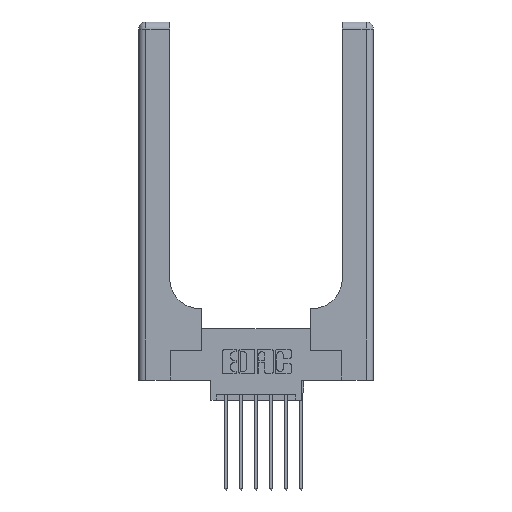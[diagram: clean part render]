
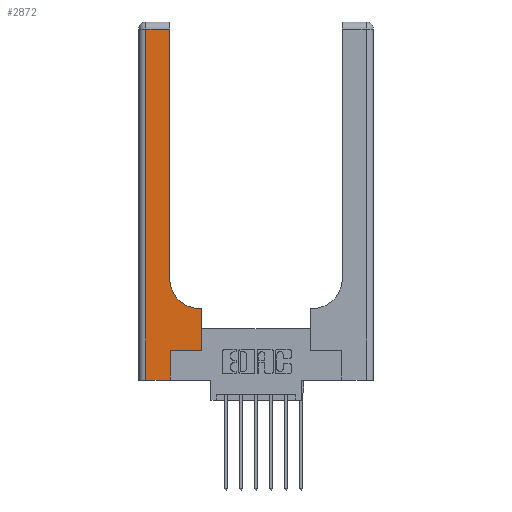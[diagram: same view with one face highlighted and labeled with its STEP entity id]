
A CAD part, top view. The second image highlights one B-rep face of the part: STEP entity #2872.
In plain terms, the highlighted planar face has unit normal (0, 0, 1).
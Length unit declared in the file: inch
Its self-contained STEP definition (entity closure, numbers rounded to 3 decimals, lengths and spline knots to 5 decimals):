
#15 = ORIENTED_EDGE ( 'NONE', *, *, #273, .T. ) ;
#273 = EDGE_CURVE ( 'NONE', #9280, #6992, #13074, .T. ) ;
#305 = AXIS2_PLACEMENT_3D ( 'NONE', #10387, #13940, #13862 ) ;
#487 = ORIENTED_EDGE ( 'NONE', *, *, #3870, .T. ) ;
#615 = LINE ( 'NONE', #5942, #1135 ) ;
#1119 = VERTEX_POINT ( 'NONE', #5577 ) ;
#1135 = VECTOR ( 'NONE', #10319, 39.37008 ) ;
#1679 = LINE ( 'NONE', #11591, #10200 ) ;
#1754 = VECTOR ( 'NONE', #6185, 39.37008 ) ;
#2082 = CARTESIAN_POINT ( 'NONE',  ( 0., 2.94, 0.37 ) ) ;
#2100 = DIRECTION ( 'NONE',  ( 1., 0., 0. ) ) ;
#2111 = CARTESIAN_POINT ( 'NONE',  ( 0.265, 0., 0.37 ) ) ;
#2166 = EDGE_CURVE ( 'NONE', #2642, #12599, #1679, .T. ) ;
#2642 = VERTEX_POINT ( 'NONE', #14012 ) ;
#2648 = VECTOR ( 'NONE', #4425, 39.37008 ) ;
#2872 = ADVANCED_FACE ( 'NONE', ( #6914 ), #4704, .F. ) ;
#2896 = AXIS2_PLACEMENT_3D ( 'NONE', #3637, #11289, #4423 ) ;
#3637 = CARTESIAN_POINT ( 'NONE',  ( 0., 3., 0.37 ) ) ;
#3650 = ORIENTED_EDGE ( 'NONE', *, *, #7391, .T. ) ;
#3870 = EDGE_CURVE ( 'NONE', #4499, #9280, #8801, .T. ) ;
#4423 = DIRECTION ( 'NONE',  ( -1., 0., 0. ) ) ;
#4425 = DIRECTION ( 'NONE',  ( -1., 0., 0. ) ) ;
#4499 = VERTEX_POINT ( 'NONE', #10076 ) ;
#4564 = EDGE_CURVE ( 'NONE', #12599, #7520, #9417, .T. ) ;
#4704 = PLANE ( 'NONE',  #2896 ) ;
#4987 = CARTESIAN_POINT ( 'NONE',  ( 0.06, 2.94, 0.37 ) ) ;
#5164 = CARTESIAN_POINT ( 'NONE',  ( 0., 0., 0.37 ) ) ;
#5577 = CARTESIAN_POINT ( 'NONE',  ( 0.51, 0.6, 0.37 ) ) ;
#5881 = CARTESIAN_POINT ( 'NONE',  ( 0.06, 0., 0.37 ) ) ;
#5942 = CARTESIAN_POINT ( 'NONE',  ( 0.26, 3., 0.37 ) ) ;
#6185 = DIRECTION ( 'NONE',  ( 0., 1., 0. ) ) ;
#6188 = LINE ( 'NONE', #7118, #6389 ) ;
#6356 = CARTESIAN_POINT ( 'NONE',  ( 0.26, 0.85, 0.37 ) ) ;
#6359 = CARTESIAN_POINT ( 'NONE',  ( 0.528, 0.6, 0.37 ) ) ;
#6389 = VECTOR ( 'NONE', #8336, 39.37008 ) ;
#6428 = CIRCLE ( 'NONE', #305, 0.25 ) ;
#6914 = FACE_OUTER_BOUND ( 'NONE', #9129, .T. ) ;
#6992 = VERTEX_POINT ( 'NONE', #5881 ) ;
#7118 = CARTESIAN_POINT ( 'NONE',  ( 0.26, 0.6, 0.37 ) ) ;
#7391 = EDGE_CURVE ( 'NONE', #13754, #4499, #615, .T. ) ;
#7520 = VERTEX_POINT ( 'NONE', #6359 ) ;
#7649 = EDGE_CURVE ( 'NONE', #13379, #2642, #9729, .T. ) ;
#8278 = EDGE_CURVE ( 'NONE', #6992, #13379, #11673, .T. ) ;
#8336 = DIRECTION ( 'NONE',  ( -1., 0., 0. ) ) ;
#8801 = LINE ( 'NONE', #2082, #2648 ) ;
#9129 = EDGE_LOOP ( 'NONE', ( #3650, #487, #15, #13179, #10462, #10946, #13648, #10937, #11899 ) ) ;
#9280 = VERTEX_POINT ( 'NONE', #4987 ) ;
#9417 = LINE ( 'NONE', #12411, #1754 ) ;
#9571 = VECTOR ( 'NONE', #9949, 39.37008 ) ;
#9729 = LINE ( 'NONE', #13019, #9571 ) ;
#9949 = DIRECTION ( 'NONE',  ( 0., 1., 0. ) ) ;
#10076 = CARTESIAN_POINT ( 'NONE',  ( 0.26, 2.94, 0.37 ) ) ;
#10200 = VECTOR ( 'NONE', #12539, 39.37008 ) ;
#10319 = DIRECTION ( 'NONE',  ( 0., 1., 0. ) ) ;
#10387 = CARTESIAN_POINT ( 'NONE',  ( 0.51, 0.85, 0.37 ) ) ;
#10462 = ORIENTED_EDGE ( 'NONE', *, *, #7649, .T. ) ;
#10686 = EDGE_CURVE ( 'NONE', #7520, #1119, #6188, .T. ) ;
#10937 = ORIENTED_EDGE ( 'NONE', *, *, #10686, .T. ) ;
#10946 = ORIENTED_EDGE ( 'NONE', *, *, #2166, .T. ) ;
#11289 = DIRECTION ( 'NONE',  ( 0., 0., -1. ) ) ;
#11506 = CARTESIAN_POINT ( 'NONE',  ( 0.528, 0.25, 0.37 ) ) ;
#11591 = CARTESIAN_POINT ( 'NONE',  ( 0.265, 0.25, 0.37 ) ) ;
#11673 = LINE ( 'NONE', #5164, #12080 ) ;
#11899 = ORIENTED_EDGE ( 'NONE', *, *, #12563, .T. ) ;
#12080 = VECTOR ( 'NONE', #2100, 39.37008 ) ;
#12411 = CARTESIAN_POINT ( 'NONE',  ( 0.528, 0.25, 0.37 ) ) ;
#12539 = DIRECTION ( 'NONE',  ( 1., 0., 0. ) ) ;
#12563 = EDGE_CURVE ( 'NONE', #1119, #13754, #6428, .T. ) ;
#12599 = VERTEX_POINT ( 'NONE', #11506 ) ;
#13019 = CARTESIAN_POINT ( 'NONE',  ( 0.265, 0., 0.37 ) ) ;
#13074 = LINE ( 'NONE', #13288, #14046 ) ;
#13179 = ORIENTED_EDGE ( 'NONE', *, *, #8278, .T. ) ;
#13212 = DIRECTION ( 'NONE',  ( 0., -1., 0. ) ) ;
#13288 = CARTESIAN_POINT ( 'NONE',  ( 0.06, 3., 0.37 ) ) ;
#13379 = VERTEX_POINT ( 'NONE', #2111 ) ;
#13648 = ORIENTED_EDGE ( 'NONE', *, *, #4564, .T. ) ;
#13754 = VERTEX_POINT ( 'NONE', #6356 ) ;
#13862 = DIRECTION ( 'NONE',  ( 1., 0., 0. ) ) ;
#13940 = DIRECTION ( 'NONE',  ( 0., 0., -1. ) ) ;
#14012 = CARTESIAN_POINT ( 'NONE',  ( 0.265, 0.25, 0.37 ) ) ;
#14046 = VECTOR ( 'NONE', #13212, 39.37008 ) ;
